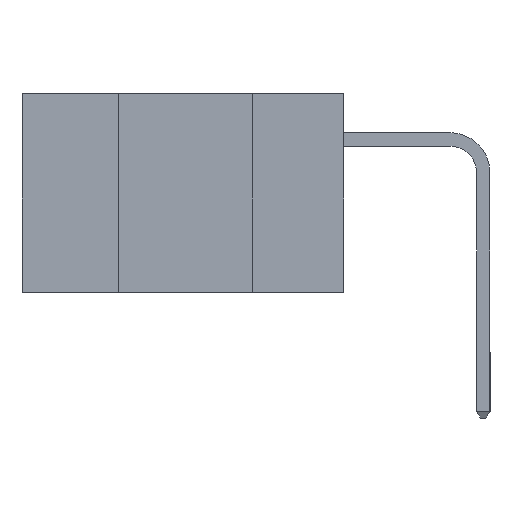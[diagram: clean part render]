
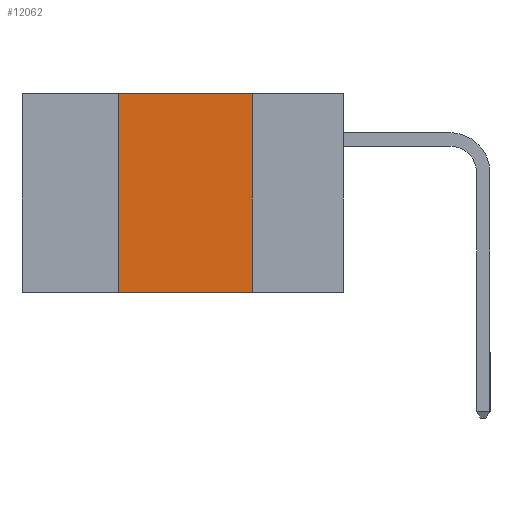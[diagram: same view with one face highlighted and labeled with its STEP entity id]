
A CAD part, left-side view. The second image highlights one B-rep face of the part: STEP entity #12062.
In plain terms, the highlighted planar face has unit normal (-1, 0, 0).
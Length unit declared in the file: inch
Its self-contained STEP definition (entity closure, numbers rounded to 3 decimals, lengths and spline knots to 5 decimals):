
#414 = PLANE ( 'NONE',  #5726 ) ;
#466 = ORIENTED_EDGE ( 'NONE', *, *, #8575, .T. ) ;
#813 = LINE ( 'NONE', #889, #12313 ) ;
#889 = CARTESIAN_POINT ( 'NONE',  ( 0., 0.42, -0.37 ) ) ;
#1912 = LINE ( 'NONE', #7365, #1967 ) ;
#1967 = VECTOR ( 'NONE', #9301, 39.37008 ) ;
#2628 = VERTEX_POINT ( 'NONE', #13270 ) ;
#3252 = VECTOR ( 'NONE', #7308, 39.37008 ) ;
#3695 = VECTOR ( 'NONE', #6399, 39.37008 ) ;
#3791 = EDGE_LOOP ( 'NONE', ( #7494, #8906, #7713, #466 ) ) ;
#3916 = CARTESIAN_POINT ( 'NONE',  ( 0., 0.6, 0. ) ) ;
#4420 = DIRECTION ( 'NONE',  ( 1., 0., 0. ) ) ;
#5726 = AXIS2_PLACEMENT_3D ( 'NONE', #7599, #4420, #6498 ) ;
#6116 = DIRECTION ( 'NONE',  ( 0., 0., 1. ) ) ;
#6399 = DIRECTION ( 'NONE',  ( 0., 0., -1. ) ) ;
#6498 = DIRECTION ( 'NONE',  ( 0., 0., -1. ) ) ;
#6908 = CARTESIAN_POINT ( 'NONE',  ( 0., 0.42, 0. ) ) ;
#7173 = EDGE_CURVE ( 'NONE', #12183, #2628, #11498, .T. ) ;
#7308 = DIRECTION ( 'NONE',  ( 0., -1., 0. ) ) ;
#7365 = CARTESIAN_POINT ( 'NONE',  ( 0., 0.6, -0.37 ) ) ;
#7391 = EDGE_CURVE ( 'NONE', #2628, #10064, #9431, .T. ) ;
#7409 = CARTESIAN_POINT ( 'NONE',  ( 0., 0.17, -0.37 ) ) ;
#7494 = ORIENTED_EDGE ( 'NONE', *, *, #7391, .F. ) ;
#7599 = CARTESIAN_POINT ( 'NONE',  ( 0., 0.6, 0. ) ) ;
#7713 = ORIENTED_EDGE ( 'NONE', *, *, #11399, .F. ) ;
#8122 = VERTEX_POINT ( 'NONE', #9718 ) ;
#8575 = EDGE_CURVE ( 'NONE', #8122, #10064, #1912, .T. ) ;
#8906 = ORIENTED_EDGE ( 'NONE', *, *, #7173, .F. ) ;
#9301 = DIRECTION ( 'NONE',  ( 0., -1., 0. ) ) ;
#9431 = LINE ( 'NONE', #9701, #3695 ) ;
#9701 = CARTESIAN_POINT ( 'NONE',  ( 0., 0.17, -0.37 ) ) ;
#9718 = CARTESIAN_POINT ( 'NONE',  ( 0., 0.42, -0.37 ) ) ;
#10064 = VERTEX_POINT ( 'NONE', #7409 ) ;
#11399 = EDGE_CURVE ( 'NONE', #8122, #12183, #813, .T. ) ;
#11498 = LINE ( 'NONE', #3916, #3252 ) ;
#11653 = FACE_OUTER_BOUND ( 'NONE', #3791, .T. ) ;
#12062 = ADVANCED_FACE ( 'NONE', ( #11653 ), #414, .F. ) ;
#12183 = VERTEX_POINT ( 'NONE', #6908 ) ;
#12313 = VECTOR ( 'NONE', #6116, 39.37008 ) ;
#13270 = CARTESIAN_POINT ( 'NONE',  ( 0., 0.17, 0. ) ) ;
